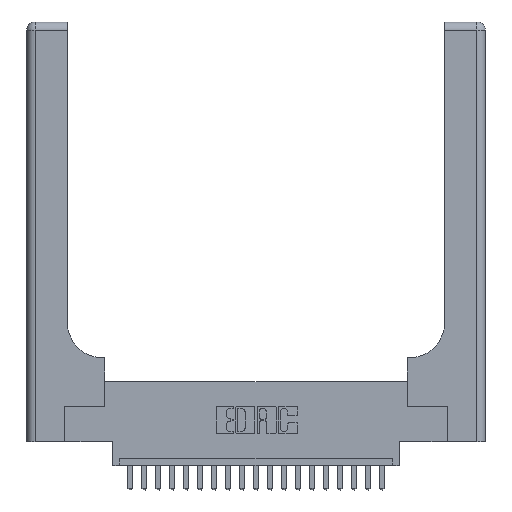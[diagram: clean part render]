
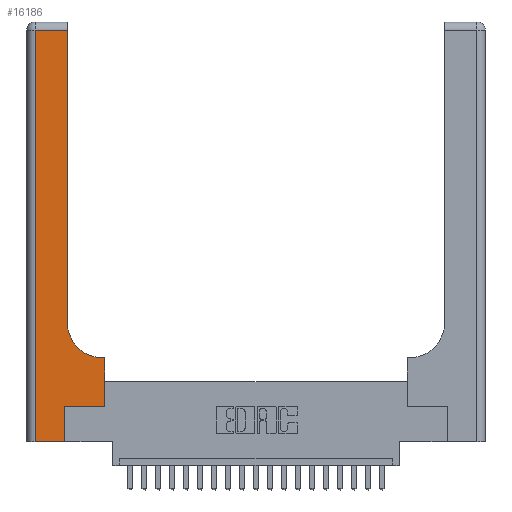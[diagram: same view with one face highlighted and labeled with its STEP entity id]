
A CAD part, top view. The second image highlights one B-rep face of the part: STEP entity #16186.
In plain terms, the highlighted planar face has unit normal (0, 0, 1).
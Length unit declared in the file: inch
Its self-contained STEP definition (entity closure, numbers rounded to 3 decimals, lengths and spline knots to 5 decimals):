
#360 = CARTESIAN_POINT ( 'NONE',  ( 0.5585, 0.6, 0.37 ) ) ;
#412 = DIRECTION ( 'NONE',  ( -1., 0., 0. ) ) ;
#548 = AXIS2_PLACEMENT_3D ( 'NONE', #22291, #20989, #13384 ) ;
#566 = CARTESIAN_POINT ( 'NONE',  ( 0., 3., 0.37 ) ) ;
#909 = VERTEX_POINT ( 'NONE', #4342 ) ;
#1176 = EDGE_CURVE ( 'NONE', #2869, #17615, #6161, .T. ) ;
#1483 = ORIENTED_EDGE ( 'NONE', *, *, #14343, .T. ) ;
#1530 = VERTEX_POINT ( 'NONE', #14371 ) ;
#1654 = LINE ( 'NONE', #18795, #19843 ) ;
#2130 = VECTOR ( 'NONE', #7689, 39.37008 ) ;
#2826 = CARTESIAN_POINT ( 'NONE',  ( 0.2915, 0.85, 0.37 ) ) ;
#2869 = VERTEX_POINT ( 'NONE', #360 ) ;
#3096 = CARTESIAN_POINT ( 'NONE',  ( 0.269, 0.25, 0.37 ) ) ;
#3102 = VECTOR ( 'NONE', #11950, 39.37008 ) ;
#3297 = VERTEX_POINT ( 'NONE', #14010 ) ;
#4090 = EDGE_CURVE ( 'NONE', #3297, #1530, #17047, .T. ) ;
#4342 = CARTESIAN_POINT ( 'NONE',  ( 0.06, 2.94, 0.37 ) ) ;
#5853 = CARTESIAN_POINT ( 'NONE',  ( 0.269, 0., 0.37 ) ) ;
#5910 = EDGE_CURVE ( 'NONE', #17968, #2869, #18610, .T. ) ;
#6161 = LINE ( 'NONE', #7936, #6958 ) ;
#6777 = VERTEX_POINT ( 'NONE', #22226 ) ;
#6958 = VECTOR ( 'NONE', #9607, 39.37008 ) ;
#7168 = CIRCLE ( 'NONE', #548, 0.25 ) ;
#7621 = ORIENTED_EDGE ( 'NONE', *, *, #11307, .T. ) ;
#7689 = DIRECTION ( 'NONE',  ( 0., 1., 0. ) ) ;
#7858 = ORIENTED_EDGE ( 'NONE', *, *, #5910, .T. ) ;
#7936 = CARTESIAN_POINT ( 'NONE',  ( 0.2915, 0.6, 0.37 ) ) ;
#8772 = VECTOR ( 'NONE', #10053, 39.37008 ) ;
#8862 = LINE ( 'NONE', #22463, #3102 ) ;
#9223 = EDGE_CURVE ( 'NONE', #6777, #909, #1654, .T. ) ;
#9320 = ORIENTED_EDGE ( 'NONE', *, *, #1176, .T. ) ;
#9352 = EDGE_CURVE ( 'NONE', #909, #9892, #22850, .T. ) ;
#9414 = DIRECTION ( 'NONE',  ( -1., 0., 0. ) ) ;
#9607 = DIRECTION ( 'NONE',  ( -1., 0., 0. ) ) ;
#9892 = VERTEX_POINT ( 'NONE', #15145 ) ;
#10053 = DIRECTION ( 'NONE',  ( 0., -1., 0. ) ) ;
#10087 = DIRECTION ( 'NONE',  ( 1., 0., 0. ) ) ;
#10130 = CARTESIAN_POINT ( 'NONE',  ( 0.06, 3., 0.37 ) ) ;
#10270 = DIRECTION ( 'NONE',  ( 0., 1., 0. ) ) ;
#10659 = AXIS2_PLACEMENT_3D ( 'NONE', #566, #21532, #412 ) ;
#11194 = FACE_OUTER_BOUND ( 'NONE', #22713, .T. ) ;
#11307 = EDGE_CURVE ( 'NONE', #9892, #3297, #8862, .T. ) ;
#11950 = DIRECTION ( 'NONE',  ( 1., 0., 0. ) ) ;
#12864 = DIRECTION ( 'NONE',  ( 0., 1., 0. ) ) ;
#13228 = LINE ( 'NONE', #3096, #17614 ) ;
#13384 = DIRECTION ( 'NONE',  ( 1., 0., 0. ) ) ;
#13934 = CARTESIAN_POINT ( 'NONE',  ( 0.5415, 0.6, 0.37 ) ) ;
#13992 = LINE ( 'NONE', #18418, #20028 ) ;
#14010 = CARTESIAN_POINT ( 'NONE',  ( 0.269, 0., 0.37 ) ) ;
#14343 = EDGE_CURVE ( 'NONE', #17517, #6777, #13992, .T. ) ;
#14371 = CARTESIAN_POINT ( 'NONE',  ( 0.269, 0.25, 0.37 ) ) ;
#15145 = CARTESIAN_POINT ( 'NONE',  ( 0.06, 0., 0.37 ) ) ;
#16118 = VECTOR ( 'NONE', #10270, 39.37008 ) ;
#16155 = PLANE ( 'NONE',  #10659 ) ;
#16186 = ADVANCED_FACE ( 'NONE', ( #11194 ), #16155, .F. ) ;
#16367 = CARTESIAN_POINT ( 'NONE',  ( 0.5585, 0.25, 0.37 ) ) ;
#16964 = EDGE_CURVE ( 'NONE', #1530, #17968, #13228, .T. ) ;
#16965 = ORIENTED_EDGE ( 'NONE', *, *, #16964, .T. ) ;
#17047 = LINE ( 'NONE', #5853, #2130 ) ;
#17517 = VERTEX_POINT ( 'NONE', #2826 ) ;
#17614 = VECTOR ( 'NONE', #10087, 39.37008 ) ;
#17615 = VERTEX_POINT ( 'NONE', #13934 ) ;
#17968 = VERTEX_POINT ( 'NONE', #16367 ) ;
#18272 = ORIENTED_EDGE ( 'NONE', *, *, #9352, .T. ) ;
#18418 = CARTESIAN_POINT ( 'NONE',  ( 0.2915, 3., 0.37 ) ) ;
#18610 = LINE ( 'NONE', #19080, #16118 ) ;
#18795 = CARTESIAN_POINT ( 'NONE',  ( 0., 2.94, 0.37 ) ) ;
#18807 = ORIENTED_EDGE ( 'NONE', *, *, #4090, .T. ) ;
#19080 = CARTESIAN_POINT ( 'NONE',  ( 0.5585, 0.25, 0.37 ) ) ;
#19397 = ORIENTED_EDGE ( 'NONE', *, *, #22180, .T. ) ;
#19843 = VECTOR ( 'NONE', #9414, 39.37008 ) ;
#20028 = VECTOR ( 'NONE', #12864, 39.37008 ) ;
#20989 = DIRECTION ( 'NONE',  ( 0., 0., -1. ) ) ;
#21288 = ORIENTED_EDGE ( 'NONE', *, *, #9223, .T. ) ;
#21532 = DIRECTION ( 'NONE',  ( 0., 0., -1. ) ) ;
#22180 = EDGE_CURVE ( 'NONE', #17615, #17517, #7168, .T. ) ;
#22226 = CARTESIAN_POINT ( 'NONE',  ( 0.2915, 2.94, 0.37 ) ) ;
#22291 = CARTESIAN_POINT ( 'NONE',  ( 0.5415, 0.85, 0.37 ) ) ;
#22463 = CARTESIAN_POINT ( 'NONE',  ( 0., 0., 0.37 ) ) ;
#22713 = EDGE_LOOP ( 'NONE', ( #1483, #21288, #18272, #7621, #18807, #16965, #7858, #9320, #19397 ) ) ;
#22850 = LINE ( 'NONE', #10130, #8772 ) ;
